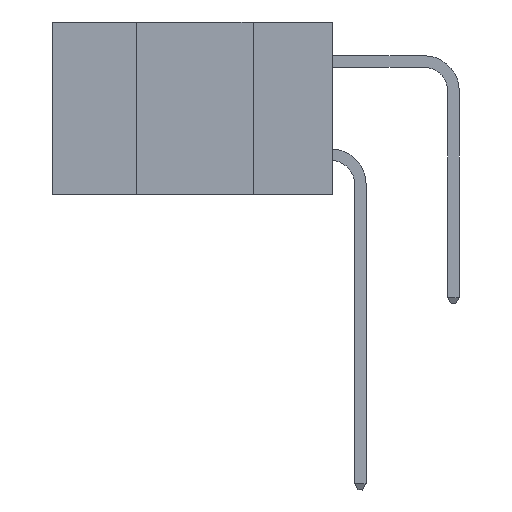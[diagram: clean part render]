
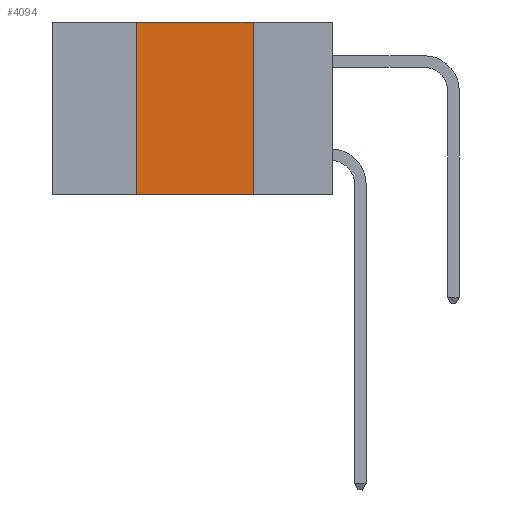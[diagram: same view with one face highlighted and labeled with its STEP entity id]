
A CAD part, left-side view. The second image highlights one B-rep face of the part: STEP entity #4094.
In plain terms, the highlighted planar face has unit normal (-1, 0, 0).
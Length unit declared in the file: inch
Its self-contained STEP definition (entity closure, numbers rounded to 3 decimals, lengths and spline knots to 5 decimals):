
#674 = DIRECTION ( 'NONE',  ( 0., -1., 0. ) ) ;
#2415 = CARTESIAN_POINT ( 'NONE',  ( 0., 0.17, 0. ) ) ;
#2458 = LINE ( 'NONE', #8828, #9242 ) ;
#3265 = ORIENTED_EDGE ( 'NONE', *, *, #16114, .F. ) ;
#3426 = EDGE_LOOP ( 'NONE', ( #19657, #3265, #17213, #17080 ) ) ;
#3552 = LINE ( 'NONE', #16568, #17887 ) ;
#3683 = CARTESIAN_POINT ( 'NONE',  ( 0., 0.17, -0.37 ) ) ;
#3708 = CARTESIAN_POINT ( 'NONE',  ( 0., 0.6, -0.37 ) ) ;
#4094 = ADVANCED_FACE ( 'NONE', ( #12247 ), #5833, .F. ) ;
#4236 = VECTOR ( 'NONE', #674, 39.37008 ) ;
#5833 = PLANE ( 'NONE',  #15797 ) ;
#6225 = DIRECTION ( 'NONE',  ( 0., -1., 0. ) ) ;
#6735 = LINE ( 'NONE', #3708, #4236 ) ;
#6951 = CARTESIAN_POINT ( 'NONE',  ( 0., 0.42, 0. ) ) ;
#7253 = DIRECTION ( 'NONE',  ( 0., 0., 1. ) ) ;
#8434 = EDGE_CURVE ( 'NONE', #20068, #11838, #3552, .T. ) ;
#8828 = CARTESIAN_POINT ( 'NONE',  ( 0., 0.42, -0.37 ) ) ;
#9242 = VECTOR ( 'NONE', #7253, 39.37008 ) ;
#9929 = DIRECTION ( 'NONE',  ( 0., 0., -1. ) ) ;
#11455 = EDGE_CURVE ( 'NONE', #11720, #11838, #6735, .T. ) ;
#11720 = VERTEX_POINT ( 'NONE', #12615 ) ;
#11838 = VERTEX_POINT ( 'NONE', #3683 ) ;
#12247 = FACE_OUTER_BOUND ( 'NONE', #3426, .T. ) ;
#12352 = CARTESIAN_POINT ( 'NONE',  ( 0., 0.6, 0. ) ) ;
#12615 = CARTESIAN_POINT ( 'NONE',  ( 0., 0.42, -0.37 ) ) ;
#12751 = CARTESIAN_POINT ( 'NONE',  ( 0., 0.6, 0. ) ) ;
#14018 = VECTOR ( 'NONE', #6225, 39.37008 ) ;
#15797 = AXIS2_PLACEMENT_3D ( 'NONE', #12352, #18769, #17498 ) ;
#16114 = EDGE_CURVE ( 'NONE', #19059, #20068, #20638, .T. ) ;
#16568 = CARTESIAN_POINT ( 'NONE',  ( 0., 0.17, -0.37 ) ) ;
#17080 = ORIENTED_EDGE ( 'NONE', *, *, #11455, .T. ) ;
#17213 = ORIENTED_EDGE ( 'NONE', *, *, #19195, .F. ) ;
#17498 = DIRECTION ( 'NONE',  ( 0., 0., -1. ) ) ;
#17887 = VECTOR ( 'NONE', #9929, 39.37008 ) ;
#18769 = DIRECTION ( 'NONE',  ( 1., 0., 0. ) ) ;
#19059 = VERTEX_POINT ( 'NONE', #6951 ) ;
#19195 = EDGE_CURVE ( 'NONE', #11720, #19059, #2458, .T. ) ;
#19657 = ORIENTED_EDGE ( 'NONE', *, *, #8434, .F. ) ;
#20068 = VERTEX_POINT ( 'NONE', #2415 ) ;
#20638 = LINE ( 'NONE', #12751, #14018 ) ;
